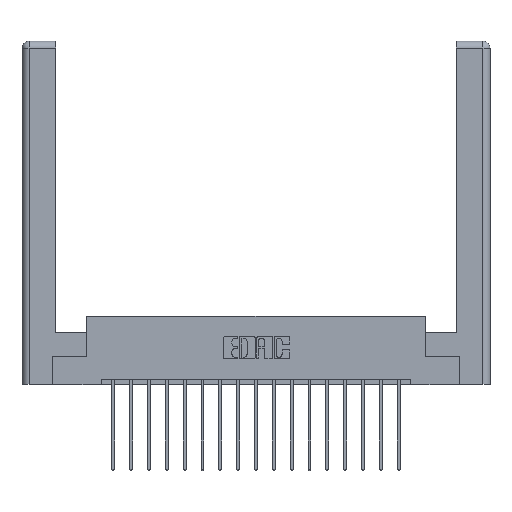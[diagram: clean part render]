
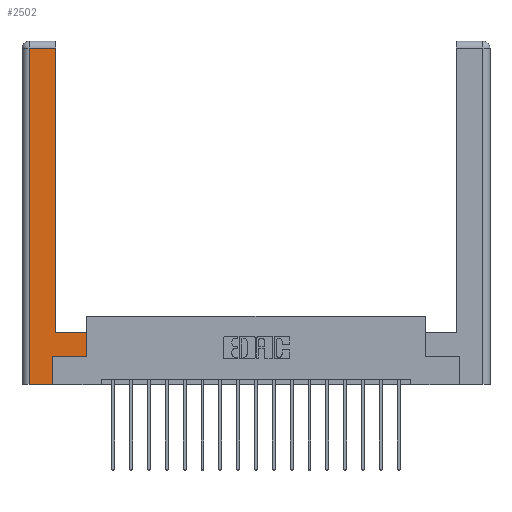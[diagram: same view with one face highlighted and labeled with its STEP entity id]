
A CAD part, top view. The second image highlights one B-rep face of the part: STEP entity #2502.
In plain terms, the highlighted planar face has unit normal (0, 0, 1).
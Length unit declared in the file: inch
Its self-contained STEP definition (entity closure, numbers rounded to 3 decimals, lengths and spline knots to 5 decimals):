
#475 = DIRECTION ( 'NONE',  ( 1., 0., 0. ) ) ;
#543 = EDGE_LOOP ( 'NONE', ( #18754, #6816, #15026, #13086, #2260, #4495, #10858, #12552 ) ) ;
#567 = CARTESIAN_POINT ( 'NONE',  ( 0., 0., 0. ) ) ;
#594 = LINE ( 'NONE', #12919, #15561 ) ;
#603 = EDGE_CURVE ( 'NONE', #13508, #7165, #1863, .T. ) ;
#1301 = AXIS2_PLACEMENT_3D ( 'NONE', #567, #9308, #7936 ) ;
#1410 = EDGE_CURVE ( 'NONE', #4059, #13508, #11759, .T. ) ;
#1863 = LINE ( 'NONE', #3365, #15687 ) ;
#2119 = DIRECTION ( 'NONE',  ( 0., 1., 0. ) ) ;
#2217 = CARTESIAN_POINT ( 'NONE',  ( 0.295, 2.94, 0. ) ) ;
#2260 = ORIENTED_EDGE ( 'NONE', *, *, #11925, .T. ) ;
#2502 = ADVANCED_FACE ( 'NONE', ( #12151 ), #16646, .F. ) ;
#2605 = EDGE_CURVE ( 'NONE', #10976, #4059, #8441, .T. ) ;
#2658 = CARTESIAN_POINT ( 'NONE',  ( 0.565, 0.245, 0. ) ) ;
#2889 = CARTESIAN_POINT ( 'NONE',  ( 0.265, 0., 0. ) ) ;
#3227 = CARTESIAN_POINT ( 'NONE',  ( 0.0615, 2.94, 0. ) ) ;
#3357 = LINE ( 'NONE', #15284, #16017 ) ;
#3365 = CARTESIAN_POINT ( 'NONE',  ( 0.0615, 2.94, 0. ) ) ;
#3677 = VECTOR ( 'NONE', #2119, 39.37008 ) ;
#4059 = VERTEX_POINT ( 'NONE', #16239 ) ;
#4495 = ORIENTED_EDGE ( 'NONE', *, *, #14047, .T. ) ;
#4767 = VERTEX_POINT ( 'NONE', #2658 ) ;
#5863 = VECTOR ( 'NONE', #14953, 39.37008 ) ;
#6255 = CARTESIAN_POINT ( 'NONE',  ( 0.565, 0.45, 0. ) ) ;
#6816 = ORIENTED_EDGE ( 'NONE', *, *, #603, .T. ) ;
#7165 = VERTEX_POINT ( 'NONE', #3227 ) ;
#7500 = VECTOR ( 'NONE', #10088, 39.37008 ) ;
#7745 = VECTOR ( 'NONE', #17158, 39.37008 ) ;
#7936 = DIRECTION ( 'NONE',  ( -1., 0., 0. ) ) ;
#8441 = LINE ( 'NONE', #13967, #7745 ) ;
#8792 = CARTESIAN_POINT ( 'NONE',  ( 0.0615, 0., 0. ) ) ;
#9308 = DIRECTION ( 'NONE',  ( 0., 0., -1. ) ) ;
#9433 = VERTEX_POINT ( 'NONE', #2889 ) ;
#9884 = EDGE_CURVE ( 'NONE', #7165, #16875, #15743, .T. ) ;
#10088 = DIRECTION ( 'NONE',  ( 0., 1., 0. ) ) ;
#10515 = DIRECTION ( 'NONE',  ( 0., 1., 0. ) ) ;
#10761 = LINE ( 'NONE', #18915, #7500 ) ;
#10858 = ORIENTED_EDGE ( 'NONE', *, *, #13747, .T. ) ;
#10908 = CARTESIAN_POINT ( 'NONE',  ( 0.295, 3., 0. ) ) ;
#10976 = VERTEX_POINT ( 'NONE', #6255 ) ;
#11759 = LINE ( 'NONE', #10908, #3677 ) ;
#11925 = EDGE_CURVE ( 'NONE', #9433, #12271, #14749, .T. ) ;
#12151 = FACE_OUTER_BOUND ( 'NONE', #543, .T. ) ;
#12271 = VERTEX_POINT ( 'NONE', #18470 ) ;
#12552 = ORIENTED_EDGE ( 'NONE', *, *, #2605, .T. ) ;
#12919 = CARTESIAN_POINT ( 'NONE',  ( 0.565, 0.245, 0. ) ) ;
#13086 = ORIENTED_EDGE ( 'NONE', *, *, #17282, .T. ) ;
#13508 = VERTEX_POINT ( 'NONE', #2217 ) ;
#13644 = DIRECTION ( 'NONE',  ( -1., 0., 0. ) ) ;
#13747 = EDGE_CURVE ( 'NONE', #4767, #10976, #10761, .T. ) ;
#13967 = CARTESIAN_POINT ( 'NONE',  ( 0.295, 0.45, 0. ) ) ;
#14047 = EDGE_CURVE ( 'NONE', #12271, #4767, #594, .T. ) ;
#14749 = LINE ( 'NONE', #14896, #17976 ) ;
#14896 = CARTESIAN_POINT ( 'NONE',  ( 0.265, 0.245, 0. ) ) ;
#14953 = DIRECTION ( 'NONE',  ( 0., -1., 0. ) ) ;
#15026 = ORIENTED_EDGE ( 'NONE', *, *, #9884, .T. ) ;
#15284 = CARTESIAN_POINT ( 'NONE',  ( 0.265, 0., 0. ) ) ;
#15561 = VECTOR ( 'NONE', #15783, 39.37008 ) ;
#15687 = VECTOR ( 'NONE', #13644, 39.37008 ) ;
#15743 = LINE ( 'NONE', #8792, #5863 ) ;
#15783 = DIRECTION ( 'NONE',  ( 1., 0., 0. ) ) ;
#16017 = VECTOR ( 'NONE', #475, 39.37008 ) ;
#16239 = CARTESIAN_POINT ( 'NONE',  ( 0.295, 0.45, 0. ) ) ;
#16646 = PLANE ( 'NONE',  #1301 ) ;
#16875 = VERTEX_POINT ( 'NONE', #17042 ) ;
#17042 = CARTESIAN_POINT ( 'NONE',  ( 0.0615, 0., 0. ) ) ;
#17158 = DIRECTION ( 'NONE',  ( -1., 0., 0. ) ) ;
#17282 = EDGE_CURVE ( 'NONE', #16875, #9433, #3357, .T. ) ;
#17976 = VECTOR ( 'NONE', #10515, 39.37008 ) ;
#18470 = CARTESIAN_POINT ( 'NONE',  ( 0.265, 0.245, 0. ) ) ;
#18754 = ORIENTED_EDGE ( 'NONE', *, *, #1410, .T. ) ;
#18915 = CARTESIAN_POINT ( 'NONE',  ( 0.565, 0.45, 0. ) ) ;
